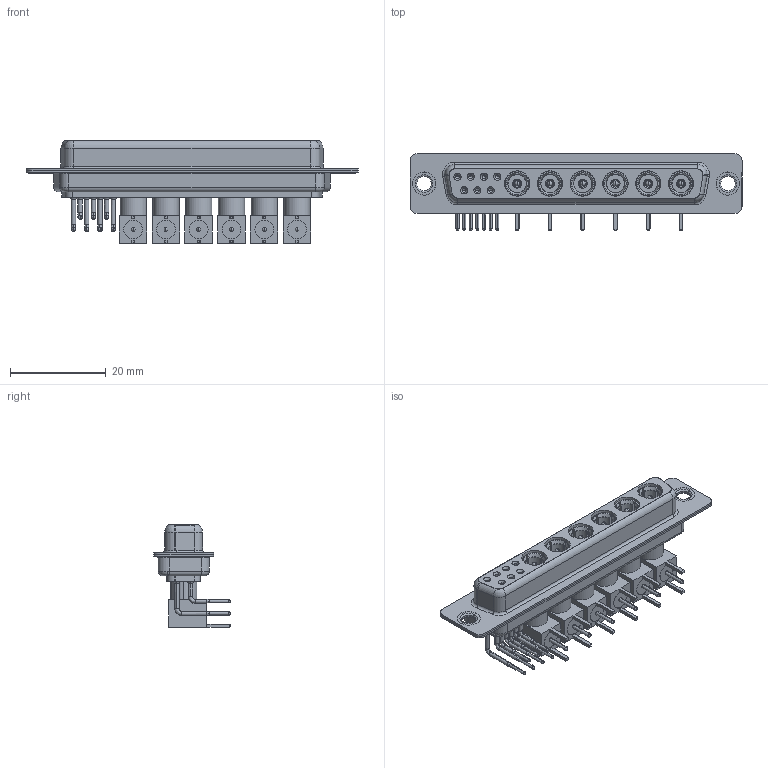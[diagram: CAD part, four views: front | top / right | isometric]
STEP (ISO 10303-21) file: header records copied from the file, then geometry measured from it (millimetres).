
FILE_DESCRIPTION (( 'STEP AP203' ), '1' );
FILE_NAME ('630-13W6240-7T1.STEP', '2022-06-03T12:49:48', ( '' ), ( '' ), 'SwSTEP 2.0', 'SolidWorks 2020', '' );
FILE_SCHEMA (( 'CONFIG_CONTROL_DESIGN' ));
Length unit declared in the file: millimetre
Products named in the file (19): Co-Ax Plug Assy_RA; Co-Ax Plug_RA PC Tail; 630Combo Contact Row 1; RA Back Shell; 630Combo Shell Rear_37 Contacts; Insulator Pin_Straight PC Tail; 630Combo Shell Front_37 Contacts; 630Combo Contact Row 2; 630Combo Thru Hole Rivet; Locking Collar; 630Combo Housing_13W6; 630-13W6240-7T1; Pin_RA; Insulator RA Pin
Assembly tree (54 placements, depth 3):
  630-13W6240-7T1
    630Combo Housing_13W6
    630Combo Shell Front_37 Contacts
    630Combo Shell Rear_37 Contacts
    630Combo Thru Hole Rivet  x2
    Co-Ax Plug Assy_RA
      Co-Ax Plug_RA PC Tail
      Insulator Pin_Straight PC Tail
      Pin_RA
      Locking Collar
      RA Back Shell
      Insulator RA Pin
    Co-Ax Plug Assy_RA
      Co-Ax Plug_RA PC Tail
      Insulator Pin_Straight PC Tail
      Pin_RA
      Locking Collar
      RA Back Shell
      Insulator RA Pin
    Co-Ax Plug Assy_RA
      Co-Ax Plug_RA PC Tail
      Insulator Pin_Straight PC Tail
      Pin_RA
      Locking Collar
      RA Back Shell
      Insulator RA Pin
    Co-Ax Plug Assy_RA
      Co-Ax Plug_RA PC Tail
      Insulator Pin_Straight PC Tail
      Pin_RA
      Locking Collar
      RA Back Shell
      Insulator RA Pin
    Co-Ax Plug Assy_RA
      Co-Ax Plug_RA PC Tail
      Insulator Pin_Straight PC Tail
      Pin_RA
      Locking Collar
      RA Back Shell
      Insulator RA Pin
    Co-Ax Plug Assy_RA
      Co-Ax Plug_RA PC Tail
      Insulator Pin_Straight PC Tail
      Pin_RA
      Locking Collar
      RA Back Shell
      Insulator RA Pin
    630Combo Contact Row 1  x4
    630Combo Contact Row 2  x3
Bounding box: 69.4 x 16 x 21.41 mm (x, y, z)
Volume: 6592.5 mm3; surface area: 15810.1 mm2
Topology: 48 solids, 48 shells, 1632 faces, 3954 edges, 2472 vertices
Faces by surface type: cylinder 672, plane 574, cone 227, torus 101, bspline 34, sphere 24
Entity records: 21068 total; most frequent: CARTESIAN_POINT 3567, DIRECTION 3361, ORIENTED_EDGE 2828, EDGE_CURVE 1414, AXIS2_PLACEMENT_3D 1383, VERTEX_POINT 896, CIRCLE 732, EDGE_LOOP 700
